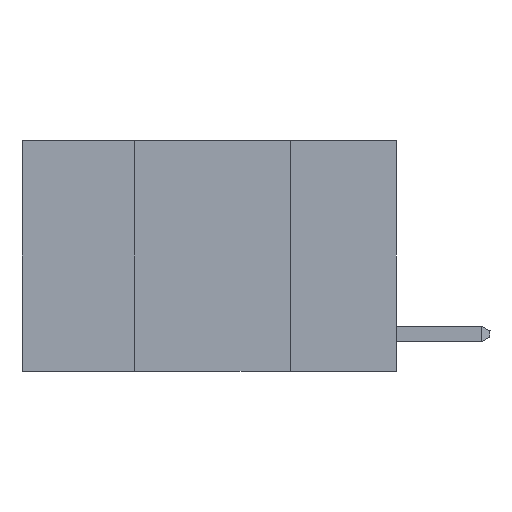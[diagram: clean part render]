
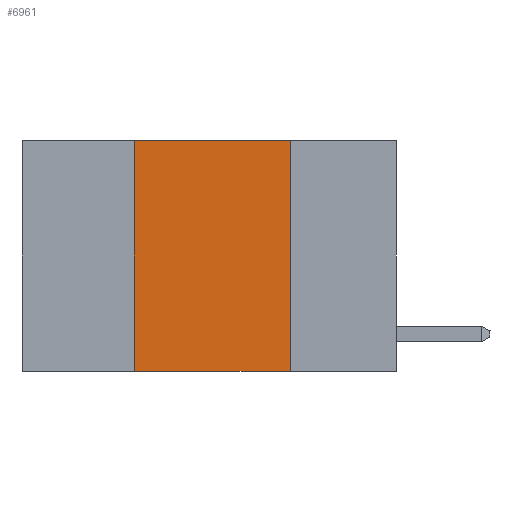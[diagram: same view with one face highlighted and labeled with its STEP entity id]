
A CAD part, left-side view. The second image highlights one B-rep face of the part: STEP entity #6961.
In plain terms, the highlighted planar face has unit normal (-1, 0, 0).
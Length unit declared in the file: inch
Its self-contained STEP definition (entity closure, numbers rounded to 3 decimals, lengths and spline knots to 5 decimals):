
#995 = CARTESIAN_POINT ( 'NONE',  ( 0., 0.42, 0. ) ) ;
#1410 = DIRECTION ( 'NONE',  ( 0., -1., 0. ) ) ;
#1673 = DIRECTION ( 'NONE',  ( 1., 0., 0. ) ) ;
#3352 = DIRECTION ( 'NONE',  ( 0., -1., 0. ) ) ;
#3461 = EDGE_LOOP ( 'NONE', ( #24434, #6381, #16067, #12881 ) ) ;
#4973 = LINE ( 'NONE', #995, #15520 ) ;
#6079 = VERTEX_POINT ( 'NONE', #26980 ) ;
#6288 = PLANE ( 'NONE',  #12846 ) ;
#6381 = ORIENTED_EDGE ( 'NONE', *, *, #17130, .F. ) ;
#6961 = ADVANCED_FACE ( 'NONE', ( #19764 ), #6288, .F. ) ;
#7884 = CARTESIAN_POINT ( 'NONE',  ( 0., 0.6, 0. ) ) ;
#8446 = VECTOR ( 'NONE', #3352, 39.37008 ) ;
#9062 = VECTOR ( 'NONE', #9490, 39.37008 ) ;
#9490 = DIRECTION ( 'NONE',  ( 0., 0., -1. ) ) ;
#9567 = LINE ( 'NONE', #7884, #27133 ) ;
#10164 = VERTEX_POINT ( 'NONE', #28893 ) ;
#10832 = DIRECTION ( 'NONE',  ( 0., 0., -1. ) ) ;
#12846 = AXIS2_PLACEMENT_3D ( 'NONE', #17313, #1673, #10832 ) ;
#12881 = ORIENTED_EDGE ( 'NONE', *, *, #17938, .T. ) ;
#13725 = CARTESIAN_POINT ( 'NONE',  ( 0., 0.17, -0.37 ) ) ;
#14197 = DIRECTION ( 'NONE',  ( 0., 0., 1. ) ) ;
#15520 = VECTOR ( 'NONE', #14197, 39.37008 ) ;
#16067 = ORIENTED_EDGE ( 'NONE', *, *, #17561, .F. ) ;
#16205 = LINE ( 'NONE', #21102, #8446 ) ;
#16577 = VERTEX_POINT ( 'NONE', #25841 ) ;
#17130 = EDGE_CURVE ( 'NONE', #16577, #6079, #9567, .T. ) ;
#17313 = CARTESIAN_POINT ( 'NONE',  ( 0., 0.6, 0. ) ) ;
#17561 = EDGE_CURVE ( 'NONE', #10164, #16577, #4973, .T. ) ;
#17938 = EDGE_CURVE ( 'NONE', #10164, #27927, #16205, .T. ) ;
#19764 = FACE_OUTER_BOUND ( 'NONE', #3461, .T. ) ;
#21102 = CARTESIAN_POINT ( 'NONE',  ( 0., 0.6, -0.37 ) ) ;
#24434 = ORIENTED_EDGE ( 'NONE', *, *, #24546, .F. ) ;
#24534 = CARTESIAN_POINT ( 'NONE',  ( 0., 0.17, 0. ) ) ;
#24546 = EDGE_CURVE ( 'NONE', #6079, #27927, #29130, .T. ) ;
#25841 = CARTESIAN_POINT ( 'NONE',  ( 0., 0.42, 0. ) ) ;
#26980 = CARTESIAN_POINT ( 'NONE',  ( 0., 0.17, 0. ) ) ;
#27133 = VECTOR ( 'NONE', #1410, 39.37008 ) ;
#27927 = VERTEX_POINT ( 'NONE', #13725 ) ;
#28893 = CARTESIAN_POINT ( 'NONE',  ( 0., 0.42, -0.37 ) ) ;
#29130 = LINE ( 'NONE', #24534, #9062 ) ;
